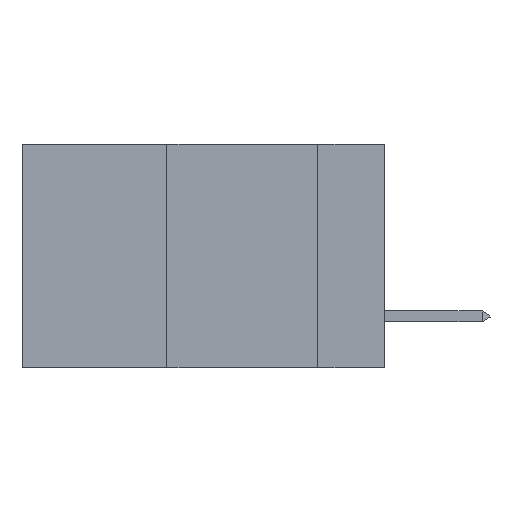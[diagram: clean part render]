
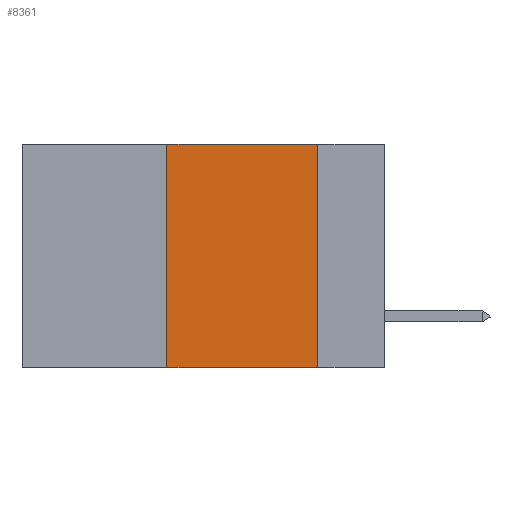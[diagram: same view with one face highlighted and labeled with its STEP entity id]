
A CAD part, left-side view. The second image highlights one B-rep face of the part: STEP entity #8361.
In plain terms, the highlighted planar face has unit normal (-1, 0, 0).
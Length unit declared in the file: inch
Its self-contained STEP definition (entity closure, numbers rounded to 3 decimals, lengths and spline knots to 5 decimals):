
#1178 = VECTOR ( 'NONE', #25951, 39.37008 ) ;
#1973 = EDGE_CURVE ( 'NONE', #20633, #10288, #6588, .T. ) ;
#2083 = VECTOR ( 'NONE', #4193, 39.37008 ) ;
#2397 = VERTEX_POINT ( 'NONE', #6379 ) ;
#2606 = VECTOR ( 'NONE', #24774, 39.37008 ) ;
#2828 = CARTESIAN_POINT ( 'NONE',  ( 0., 0.6, -0.37 ) ) ;
#4193 = DIRECTION ( 'NONE',  ( 0., 0., -1. ) ) ;
#4194 = EDGE_CURVE ( 'NONE', #2397, #10288, #22741, .T. ) ;
#4432 = EDGE_CURVE ( 'NONE', #2397, #17353, #28619, .T. ) ;
#6286 = LINE ( 'NONE', #11113, #24727 ) ;
#6379 = CARTESIAN_POINT ( 'NONE',  ( 0., 0.36, -0.37 ) ) ;
#6510 = EDGE_LOOP ( 'NONE', ( #25777, #25070, #12934, #26911 ) ) ;
#6588 = LINE ( 'NONE', #15183, #2083 ) ;
#8361 = ADVANCED_FACE ( 'NONE', ( #10145 ), #17680, .F. ) ;
#9088 = DIRECTION ( 'NONE',  ( 0., 0., -1. ) ) ;
#10145 = FACE_OUTER_BOUND ( 'NONE', #6510, .T. ) ;
#10288 = VERTEX_POINT ( 'NONE', #13304 ) ;
#10505 = CARTESIAN_POINT ( 'NONE',  ( 0., 0.11, 0. ) ) ;
#11113 = CARTESIAN_POINT ( 'NONE',  ( 0., 0.6, 0. ) ) ;
#12934 = ORIENTED_EDGE ( 'NONE', *, *, #4432, .F. ) ;
#13304 = CARTESIAN_POINT ( 'NONE',  ( 0., 0.11, -0.37 ) ) ;
#14937 = EDGE_CURVE ( 'NONE', #17353, #20633, #6286, .T. ) ;
#15183 = CARTESIAN_POINT ( 'NONE',  ( 0., 0.11, 0. ) ) ;
#17353 = VERTEX_POINT ( 'NONE', #24632 ) ;
#17680 = PLANE ( 'NONE',  #20464 ) ;
#20464 = AXIS2_PLACEMENT_3D ( 'NONE', #22417, #26609, #9088 ) ;
#20633 = VERTEX_POINT ( 'NONE', #10505 ) ;
#22417 = CARTESIAN_POINT ( 'NONE',  ( 0., 0.6, 0. ) ) ;
#22741 = LINE ( 'NONE', #2828, #2606 ) ;
#24632 = CARTESIAN_POINT ( 'NONE',  ( 0., 0.36, 0. ) ) ;
#24727 = VECTOR ( 'NONE', #28424, 39.37008 ) ;
#24774 = DIRECTION ( 'NONE',  ( 0., -1., 0. ) ) ;
#25070 = ORIENTED_EDGE ( 'NONE', *, *, #14937, .F. ) ;
#25777 = ORIENTED_EDGE ( 'NONE', *, *, #1973, .F. ) ;
#25951 = DIRECTION ( 'NONE',  ( 0., 0., 1. ) ) ;
#26609 = DIRECTION ( 'NONE',  ( 1., 0., 0. ) ) ;
#26911 = ORIENTED_EDGE ( 'NONE', *, *, #4194, .T. ) ;
#28094 = CARTESIAN_POINT ( 'NONE',  ( 0., 0.36, 0. ) ) ;
#28424 = DIRECTION ( 'NONE',  ( 0., -1., 0. ) ) ;
#28619 = LINE ( 'NONE', #28094, #1178 ) ;
